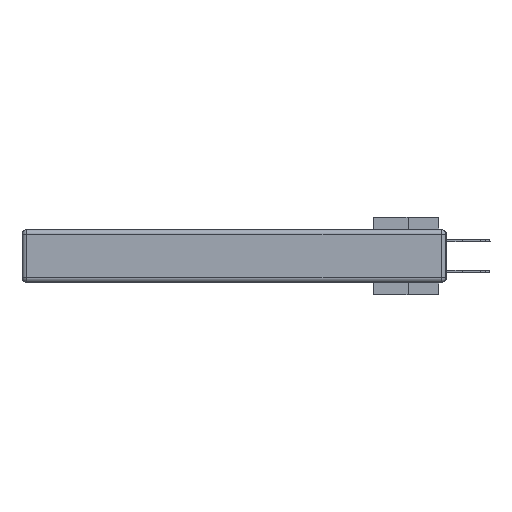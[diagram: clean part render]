
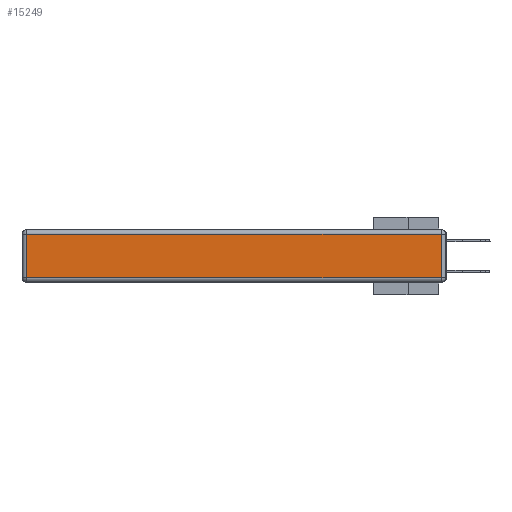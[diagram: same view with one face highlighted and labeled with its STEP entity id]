
A CAD part, left-side view. The second image highlights one B-rep face of the part: STEP entity #15249.
In plain terms, the highlighted planar face has unit normal (-1, 0, 0).
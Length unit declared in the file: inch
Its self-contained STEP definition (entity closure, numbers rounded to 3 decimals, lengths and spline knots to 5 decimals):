
#2828 = DIRECTION ( 'NONE',  ( 0., 1., 0. ) ) ;
#3458 = EDGE_CURVE ( 'NONE', #24150, #7314, #27153, .T. ) ;
#3579 = CARTESIAN_POINT ( 'NONE',  ( 0., 0., -0.343 ) ) ;
#4225 = DIRECTION ( 'NONE',  ( 0., -1., 0. ) ) ;
#4227 = EDGE_LOOP ( 'NONE', ( #12056, #13091, #20260, #24515 ) ) ;
#4768 = CARTESIAN_POINT ( 'NONE',  ( 0., 2.72, -0.343 ) ) ;
#5657 = CARTESIAN_POINT ( 'NONE',  ( 0., 0.03, -0.343 ) ) ;
#7314 = VERTEX_POINT ( 'NONE', #21379 ) ;
#8243 = VECTOR ( 'NONE', #4225, 39.37008 ) ;
#9469 = CARTESIAN_POINT ( 'NONE',  ( 0., 0.03, -0.03 ) ) ;
#10322 = EDGE_CURVE ( 'NONE', #24549, #30546, #27290, .T. ) ;
#10573 = DIRECTION ( 'NONE',  ( -1., 0., 0. ) ) ;
#12056 = ORIENTED_EDGE ( 'NONE', *, *, #10322, .T. ) ;
#13091 = ORIENTED_EDGE ( 'NONE', *, *, #16281, .T. ) ;
#14149 = LINE ( 'NONE', #4768, #18266 ) ;
#15249 = ADVANCED_FACE ( 'NONE', ( #21437 ), #20104, .T. ) ;
#16047 = CARTESIAN_POINT ( 'NONE',  ( 0., 2.75, -0.03 ) ) ;
#16281 = EDGE_CURVE ( 'NONE', #30546, #24150, #23742, .T. ) ;
#16908 = DIRECTION ( 'NONE',  ( 0., 0., -1. ) ) ;
#17580 = DIRECTION ( 'NONE',  ( 0., 0., 1. ) ) ;
#18266 = VECTOR ( 'NONE', #16908, 39.37008 ) ;
#20104 = PLANE ( 'NONE',  #28702 ) ;
#20260 = ORIENTED_EDGE ( 'NONE', *, *, #3458, .T. ) ;
#20477 = VECTOR ( 'NONE', #2828, 39.37008 ) ;
#21379 = CARTESIAN_POINT ( 'NONE',  ( 0., 2.72, -0.03 ) ) ;
#21437 = FACE_OUTER_BOUND ( 'NONE', #4227, .T. ) ;
#23173 = CARTESIAN_POINT ( 'NONE',  ( 0., 0., -0.313 ) ) ;
#23742 = LINE ( 'NONE', #5657, #24084 ) ;
#24023 = CARTESIAN_POINT ( 'NONE',  ( 0., 2.72, -0.313 ) ) ;
#24084 = VECTOR ( 'NONE', #17580, 39.37008 ) ;
#24150 = VERTEX_POINT ( 'NONE', #9469 ) ;
#24160 = EDGE_CURVE ( 'NONE', #7314, #24549, #14149, .T. ) ;
#24515 = ORIENTED_EDGE ( 'NONE', *, *, #24160, .T. ) ;
#24549 = VERTEX_POINT ( 'NONE', #24023 ) ;
#25683 = CARTESIAN_POINT ( 'NONE',  ( 0., 0.03, -0.313 ) ) ;
#27153 = LINE ( 'NONE', #16047, #20477 ) ;
#27268 = DIRECTION ( 'NONE',  ( 0., 0., 1. ) ) ;
#27290 = LINE ( 'NONE', #23173, #8243 ) ;
#28702 = AXIS2_PLACEMENT_3D ( 'NONE', #3579, #10573, #27268 ) ;
#30546 = VERTEX_POINT ( 'NONE', #25683 ) ;
